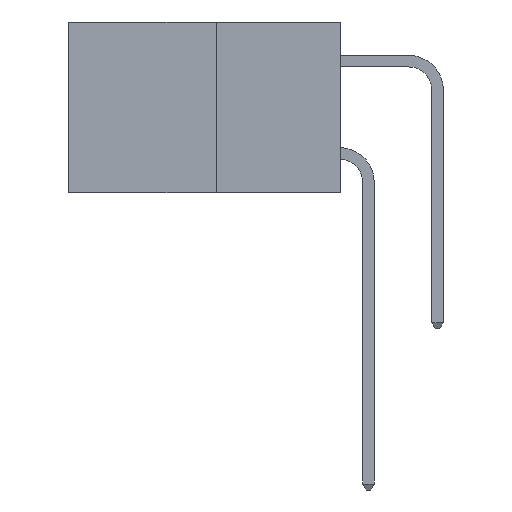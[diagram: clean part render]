
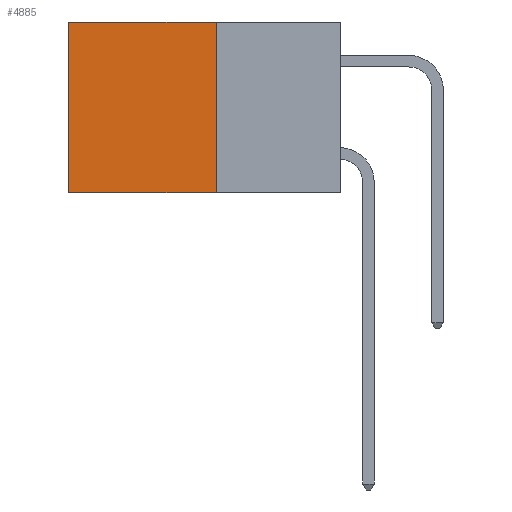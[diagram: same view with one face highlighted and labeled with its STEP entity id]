
A CAD part, left-side view. The second image highlights one B-rep face of the part: STEP entity #4885.
In plain terms, the highlighted planar face has unit normal (-1, 0, 0).
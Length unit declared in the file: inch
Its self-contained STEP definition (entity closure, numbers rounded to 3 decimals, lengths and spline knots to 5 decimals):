
#467 = ORIENTED_EDGE ( 'NONE', *, *, #553, .T. ) ;
#553 = EDGE_CURVE ( 'NONE', #9845, #30376, #26187, .T. ) ;
#655 = VECTOR ( 'NONE', #2012, 39.37008 ) ;
#1179 = VECTOR ( 'NONE', #25121, 39.37008 ) ;
#1181 = ORIENTED_EDGE ( 'NONE', *, *, #27127, .F. ) ;
#1223 = CARTESIAN_POINT ( 'NONE',  ( 0.277, 0.27, 0. ) ) ;
#2012 = DIRECTION ( 'NONE',  ( 0., 0., -1. ) ) ;
#2160 = ORIENTED_EDGE ( 'NONE', *, *, #29358, .F. ) ;
#3586 = CARTESIAN_POINT ( 'NONE',  ( 0.277, 0.59, -0.37 ) ) ;
#4885 = ADVANCED_FACE ( 'NONE', ( #7021 ), #9897, .F. ) ;
#6598 = VERTEX_POINT ( 'NONE', #3586 ) ;
#7021 = FACE_OUTER_BOUND ( 'NONE', #25106, .T. ) ;
#7443 = LINE ( 'NONE', #12991, #19670 ) ;
#9372 = DIRECTION ( 'NONE',  ( 0., 0., -1. ) ) ;
#9407 = CARTESIAN_POINT ( 'NONE',  ( 0.277, 0.59, -0.37 ) ) ;
#9579 = CARTESIAN_POINT ( 'NONE',  ( 0.277, 0.59, 0. ) ) ;
#9584 = DIRECTION ( 'NONE',  ( 1., 0., 0. ) ) ;
#9645 = CARTESIAN_POINT ( 'NONE',  ( 0.277, 0.27, -0.37 ) ) ;
#9845 = VERTEX_POINT ( 'NONE', #1223 ) ;
#9897 = PLANE ( 'NONE',  #23445 ) ;
#12097 = VECTOR ( 'NONE', #31082, 39.37008 ) ;
#12878 = LINE ( 'NONE', #23923, #12097 ) ;
#12991 = CARTESIAN_POINT ( 'NONE',  ( 0.277, 0.27, -0.37 ) ) ;
#15427 = DIRECTION ( 'NONE',  ( 0., 1., 0. ) ) ;
#19670 = VECTOR ( 'NONE', #15427, 39.37008 ) ;
#22788 = ORIENTED_EDGE ( 'NONE', *, *, #28340, .T. ) ;
#23445 = AXIS2_PLACEMENT_3D ( 'NONE', #9645, #9584, #9372 ) ;
#23923 = CARTESIAN_POINT ( 'NONE',  ( 0.277, 0.27, -0.37 ) ) ;
#24612 = CARTESIAN_POINT ( 'NONE',  ( 0.277, 0.27, 0. ) ) ;
#24787 = CARTESIAN_POINT ( 'NONE',  ( 0.277, 0.27, -0.37 ) ) ;
#25106 = EDGE_LOOP ( 'NONE', ( #22788, #2160, #1181, #467 ) ) ;
#25121 = DIRECTION ( 'NONE',  ( 0., 1., 0. ) ) ;
#26067 = VERTEX_POINT ( 'NONE', #24787 ) ;
#26187 = LINE ( 'NONE', #24612, #1179 ) ;
#27127 = EDGE_CURVE ( 'NONE', #9845, #26067, #12878, .T. ) ;
#28340 = EDGE_CURVE ( 'NONE', #30376, #6598, #31255, .T. ) ;
#29358 = EDGE_CURVE ( 'NONE', #26067, #6598, #7443, .T. ) ;
#30376 = VERTEX_POINT ( 'NONE', #9579 ) ;
#31082 = DIRECTION ( 'NONE',  ( 0., 0., -1. ) ) ;
#31255 = LINE ( 'NONE', #9407, #655 ) ;
